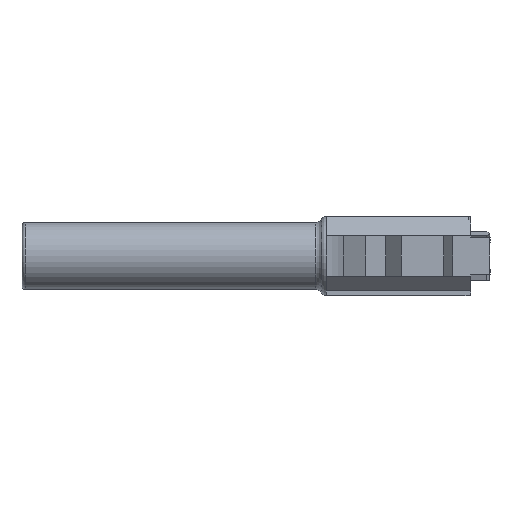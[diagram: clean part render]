
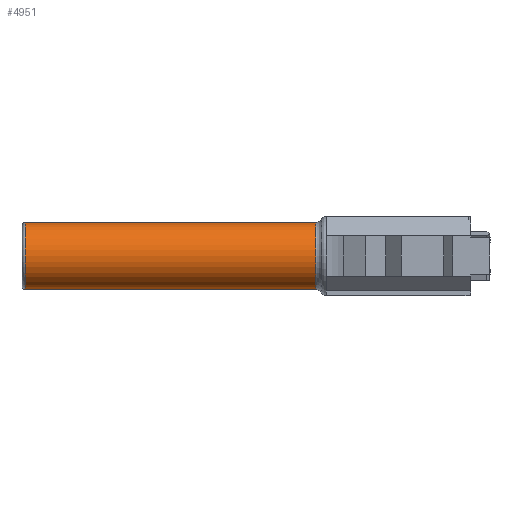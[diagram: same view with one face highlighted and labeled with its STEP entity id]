
A CAD part, front view. The second image highlights one B-rep face of the part: STEP entity #4951.
In plain terms, the highlighted cylindrical face has radius 6.991 mm (diameter 13.983 mm), a partial arc.
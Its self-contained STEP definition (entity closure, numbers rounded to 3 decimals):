
#429 = CIRCLE ( 'NONE', #7989, 6.991 ) ;
#494 = CARTESIAN_POINT ( 'NONE',  ( -17.145, -1.2, 6.991 ) ) ;
#1061 = VERTEX_POINT ( 'NONE', #3063 ) ;
#1365 = VERTEX_POINT ( 'NONE', #8516 ) ;
#1479 = LINE ( 'NONE', #2545, #5933 ) ;
#1793 = EDGE_CURVE ( 'NONE', #10774, #1061, #1479, .T. ) ;
#1867 = VECTOR ( 'NONE', #7210, 1000. ) ;
#2021 = AXIS2_PLACEMENT_3D ( 'NONE', #9436, #6939, #7789 ) ;
#2023 = FACE_OUTER_BOUND ( 'NONE', #10663, .T. ) ;
#2059 = EDGE_CURVE ( 'NONE', #4077, #1365, #4341, .T. ) ;
#2196 = EDGE_CURVE ( 'NONE', #1061, #1365, #8293, .T. ) ;
#2464 = EDGE_CURVE ( 'NONE', #4077, #10774, #429, .T. ) ;
#2545 = CARTESIAN_POINT ( 'NONE',  ( -17.145, -1.2, -6.991 ) ) ;
#2734 = ORIENTED_EDGE ( 'NONE', *, *, #2196, .F. ) ;
#2847 = DIRECTION ( 'NONE',  ( 1., 0., 0. ) ) ;
#2898 = AXIS2_PLACEMENT_3D ( 'NONE', #4927, #10804, #5764 ) ;
#3063 = CARTESIAN_POINT ( 'NONE',  ( -80.315, -1.2, -6.991 ) ) ;
#4077 = VERTEX_POINT ( 'NONE', #8538 ) ;
#4341 = LINE ( 'NONE', #494, #1867 ) ;
#4743 = CARTESIAN_POINT ( 'NONE',  ( -19.352, -1.2, -6.991 ) ) ;
#4927 = CARTESIAN_POINT ( 'NONE',  ( -80.315, -1.2, 0. ) ) ;
#4951 = ADVANCED_FACE ( 'NONE', ( #2023 ), #8201, .T. ) ;
#5764 = DIRECTION ( 'NONE',  ( 0., 0., -1. ) ) ;
#5933 = VECTOR ( 'NONE', #9264, 1000. ) ;
#6939 = DIRECTION ( 'NONE',  ( -1., 0., 0. ) ) ;
#7210 = DIRECTION ( 'NONE',  ( -1., 0., 0. ) ) ;
#7770 = ORIENTED_EDGE ( 'NONE', *, *, #2059, .T. ) ;
#7783 = ORIENTED_EDGE ( 'NONE', *, *, #2464, .F. ) ;
#7789 = DIRECTION ( 'NONE',  ( 0., 0., -1. ) ) ;
#7891 = CARTESIAN_POINT ( 'NONE',  ( -19.352, -1.2, 0. ) ) ;
#7989 = AXIS2_PLACEMENT_3D ( 'NONE', #7891, #2847, #8745 ) ;
#8201 = CYLINDRICAL_SURFACE ( 'NONE', #2021, 6.991 ) ;
#8293 = CIRCLE ( 'NONE', #2898, 6.991 ) ;
#8516 = CARTESIAN_POINT ( 'NONE',  ( -80.315, -1.2, 6.991 ) ) ;
#8538 = CARTESIAN_POINT ( 'NONE',  ( -19.352, -1.2, 6.991 ) ) ;
#8745 = DIRECTION ( 'NONE',  ( 0., 1., 0. ) ) ;
#9264 = DIRECTION ( 'NONE',  ( -1., 0., 0. ) ) ;
#9286 = ORIENTED_EDGE ( 'NONE', *, *, #1793, .F. ) ;
#9436 = CARTESIAN_POINT ( 'NONE',  ( -17.145, -1.2, 0. ) ) ;
#10663 = EDGE_LOOP ( 'NONE', ( #7783, #7770, #2734, #9286 ) ) ;
#10774 = VERTEX_POINT ( 'NONE', #4743 ) ;
#10804 = DIRECTION ( 'NONE',  ( -1., 0., 0. ) ) ;
